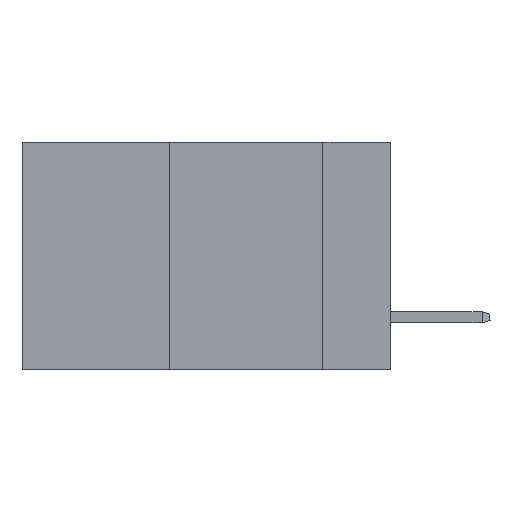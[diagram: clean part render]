
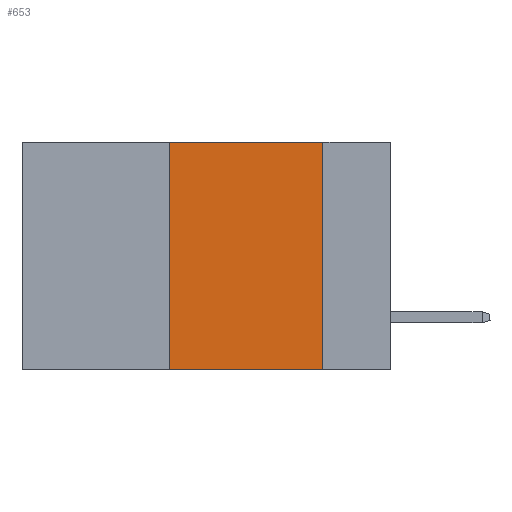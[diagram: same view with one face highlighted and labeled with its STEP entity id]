
A CAD part, left-side view. The second image highlights one B-rep face of the part: STEP entity #653.
In plain terms, the highlighted planar face has unit normal (-1, 0, 0).
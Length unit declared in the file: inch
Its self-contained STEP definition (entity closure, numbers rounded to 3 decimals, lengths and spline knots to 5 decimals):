
#29 = AXIS2_PLACEMENT_3D ( 'NONE', #12318, #24361, #29070 ) ;
#653 = ADVANCED_FACE ( 'NONE', ( #3494 ), #23564, .F. ) ;
#1810 = CARTESIAN_POINT ( 'NONE',  ( 0., 0.6, -0.37 ) ) ;
#1920 = CARTESIAN_POINT ( 'NONE',  ( 0., 0.11, 0. ) ) ;
#2939 = EDGE_CURVE ( 'NONE', #22269, #23210, #9389, .T. ) ;
#3494 = FACE_OUTER_BOUND ( 'NONE', #18230, .T. ) ;
#3604 = CARTESIAN_POINT ( 'NONE',  ( 0., 0.6, 0. ) ) ;
#5826 = DIRECTION ( 'NONE',  ( 0., -1., 0. ) ) ;
#6963 = VECTOR ( 'NONE', #5826, 39.37008 ) ;
#7496 = VECTOR ( 'NONE', #22776, 39.37008 ) ;
#8112 = ORIENTED_EDGE ( 'NONE', *, *, #2939, .F. ) ;
#8378 = CARTESIAN_POINT ( 'NONE',  ( 0., 0.11, 0. ) ) ;
#9181 = CARTESIAN_POINT ( 'NONE',  ( 0., 0.36, 0. ) ) ;
#9389 = LINE ( 'NONE', #8378, #7496 ) ;
#10834 = ORIENTED_EDGE ( 'NONE', *, *, #29415, .F. ) ;
#11229 = EDGE_CURVE ( 'NONE', #27319, #23210, #18845, .T. ) ;
#12318 = CARTESIAN_POINT ( 'NONE',  ( 0., 0.6, 0. ) ) ;
#14011 = LINE ( 'NONE', #9181, #27448 ) ;
#14657 = CARTESIAN_POINT ( 'NONE',  ( 0., 0.11, -0.37 ) ) ;
#15637 = LINE ( 'NONE', #3604, #6963 ) ;
#17370 = ORIENTED_EDGE ( 'NONE', *, *, #11229, .T. ) ;
#18230 = EDGE_LOOP ( 'NONE', ( #8112, #10834, #21097, #17370 ) ) ;
#18771 = DIRECTION ( 'NONE',  ( 0., 0., 1. ) ) ;
#18845 = LINE ( 'NONE', #1810, #23675 ) ;
#19179 = VERTEX_POINT ( 'NONE', #30750 ) ;
#21097 = ORIENTED_EDGE ( 'NONE', *, *, #23965, .F. ) ;
#22269 = VERTEX_POINT ( 'NONE', #1920 ) ;
#22776 = DIRECTION ( 'NONE',  ( 0., 0., -1. ) ) ;
#23210 = VERTEX_POINT ( 'NONE', #14657 ) ;
#23564 = PLANE ( 'NONE',  #29 ) ;
#23675 = VECTOR ( 'NONE', #25927, 39.37008 ) ;
#23965 = EDGE_CURVE ( 'NONE', #27319, #19179, #14011, .T. ) ;
#24361 = DIRECTION ( 'NONE',  ( 1., 0., 0. ) ) ;
#25927 = DIRECTION ( 'NONE',  ( 0., -1., 0. ) ) ;
#26736 = CARTESIAN_POINT ( 'NONE',  ( 0., 0.36, -0.37 ) ) ;
#27319 = VERTEX_POINT ( 'NONE', #26736 ) ;
#27448 = VECTOR ( 'NONE', #18771, 39.37008 ) ;
#29070 = DIRECTION ( 'NONE',  ( 0., 0., -1. ) ) ;
#29415 = EDGE_CURVE ( 'NONE', #19179, #22269, #15637, .T. ) ;
#30750 = CARTESIAN_POINT ( 'NONE',  ( 0., 0.36, 0. ) ) ;
